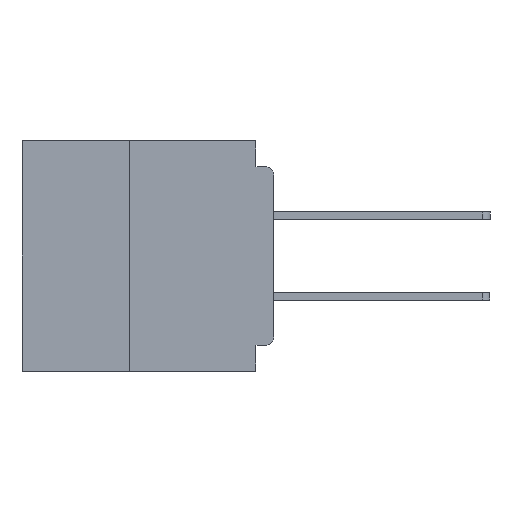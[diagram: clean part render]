
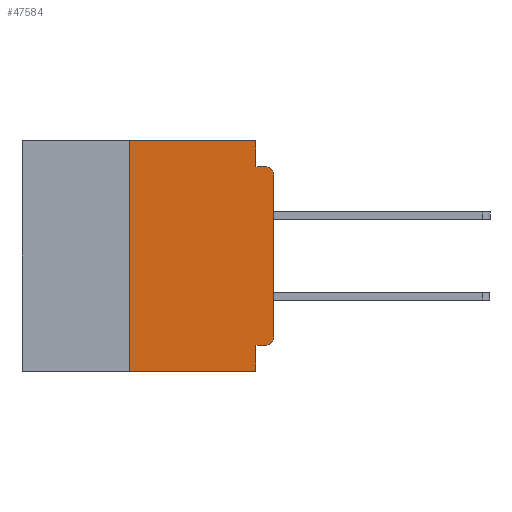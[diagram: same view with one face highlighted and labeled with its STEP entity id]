
A CAD part, left-side view. The second image highlights one B-rep face of the part: STEP entity #47584.
In plain terms, the highlighted planar face has unit normal (-1, 0, 0).
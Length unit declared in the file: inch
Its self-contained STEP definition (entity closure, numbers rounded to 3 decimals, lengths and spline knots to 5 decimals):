
#551 = ORIENTED_EDGE ( 'NONE', *, *, #44348, .F. ) ;
#1354 = CARTESIAN_POINT ( 'NONE',  ( 0., 0.015, -0.355 ) ) ;
#2596 = VERTEX_POINT ( 'NONE', #42698 ) ;
#2674 = VERTEX_POINT ( 'NONE', #37434 ) ;
#3688 = DIRECTION ( 'NONE',  ( 0., 0., -1. ) ) ;
#3971 = VECTOR ( 'NONE', #14801, 39.37008 ) ;
#4765 = CARTESIAN_POINT ( 'NONE',  ( 0., 0., 0. ) ) ;
#5240 = LINE ( 'NONE', #30179, #3971 ) ;
#5600 = CARTESIAN_POINT ( 'NONE',  ( 0., 0., -0.045 ) ) ;
#5783 = DIRECTION ( 'NONE',  ( 0., -1., 0. ) ) ;
#5863 = VECTOR ( 'NONE', #9528, 39.37008 ) ;
#6211 = ORIENTED_EDGE ( 'NONE', *, *, #15123, .T. ) ;
#8148 = EDGE_CURVE ( 'NONE', #34500, #45602, #39789, .T. ) ;
#8885 = DIRECTION ( 'NONE',  ( -1., 0., 0. ) ) ;
#9216 = EDGE_LOOP ( 'NONE', ( #45382, #16766, #22929, #38155, #13139, #35107, #6211, #551, #44868, #35758 ) ) ;
#9344 = CARTESIAN_POINT ( 'NONE',  ( 0., 0., -0.355 ) ) ;
#9528 = DIRECTION ( 'NONE',  ( 0., 1., 0. ) ) ;
#11575 = VERTEX_POINT ( 'NONE', #28146 ) ;
#13139 = ORIENTED_EDGE ( 'NONE', *, *, #25126, .F. ) ;
#14038 = VECTOR ( 'NONE', #36709, 39.37008 ) ;
#14173 = DIRECTION ( 'NONE',  ( -1., 0., 0. ) ) ;
#14774 = DIRECTION ( 'NONE',  ( 0., 0., -1. ) ) ;
#14801 = DIRECTION ( 'NONE',  ( 0., 0., 1. ) ) ;
#15123 = EDGE_CURVE ( 'NONE', #2596, #48082, #33600, .T. ) ;
#15562 = VECTOR ( 'NONE', #33870, 39.37008 ) ;
#15945 = VECTOR ( 'NONE', #5783, 39.37008 ) ;
#16476 = LINE ( 'NONE', #9344, #5863 ) ;
#16766 = ORIENTED_EDGE ( 'NONE', *, *, #32309, .T. ) ;
#17312 = VERTEX_POINT ( 'NONE', #41623 ) ;
#18422 = VERTEX_POINT ( 'NONE', #25408 ) ;
#19738 = VECTOR ( 'NONE', #40047, 39.37008 ) ;
#20898 = CARTESIAN_POINT ( 'NONE',  ( 0., 0.031, -0.045 ) ) ;
#20993 = LINE ( 'NONE', #24383, #19738 ) ;
#21926 = CARTESIAN_POINT ( 'NONE',  ( 0., 0.031, -0.355 ) ) ;
#22929 = ORIENTED_EDGE ( 'NONE', *, *, #38788, .F. ) ;
#23458 = VERTEX_POINT ( 'NONE', #20898 ) ;
#24265 = CARTESIAN_POINT ( 'NONE',  ( 0., 0., -0.34 ) ) ;
#24383 = CARTESIAN_POINT ( 'NONE',  ( 0., 0.031, -0.4 ) ) ;
#25126 = EDGE_CURVE ( 'NONE', #2674, #18422, #36331, .T. ) ;
#25408 = CARTESIAN_POINT ( 'NONE',  ( 0., 0.031, 0. ) ) ;
#26416 = CARTESIAN_POINT ( 'NONE',  ( 0., 0.437, 0. ) ) ;
#27399 = CARTESIAN_POINT ( 'NONE',  ( 0., 0.031, 0. ) ) ;
#28146 = CARTESIAN_POINT ( 'NONE',  ( 0., 0.015, -0.045 ) ) ;
#28427 = DIRECTION ( 'NONE',  ( 0., 0., 1. ) ) ;
#28882 = CARTESIAN_POINT ( 'NONE',  ( 0., 0.437, -0.4 ) ) ;
#28960 = AXIS2_PLACEMENT_3D ( 'NONE', #26416, #38172, #14774 ) ;
#29856 = CIRCLE ( 'NONE', #41732, 0.015 ) ;
#29941 = CARTESIAN_POINT ( 'NONE',  ( 0., 0.437, 0. ) ) ;
#30179 = CARTESIAN_POINT ( 'NONE',  ( 0., 0.25, -0.4 ) ) ;
#30491 = AXIS2_PLACEMENT_3D ( 'NONE', #32381, #8885, #36300 ) ;
#31690 = EDGE_CURVE ( 'NONE', #34500, #32763, #16476, .T. ) ;
#32309 = EDGE_CURVE ( 'NONE', #17312, #11575, #29856, .T. ) ;
#32381 = CARTESIAN_POINT ( 'NONE',  ( 0., 0.015, -0.34 ) ) ;
#32763 = VERTEX_POINT ( 'NONE', #21926 ) ;
#33600 = LINE ( 'NONE', #28882, #14038 ) ;
#33788 = EDGE_CURVE ( 'NONE', #45602, #17312, #47873, .T. ) ;
#33870 = DIRECTION ( 'NONE',  ( 0., -1., 0. ) ) ;
#34254 = PLANE ( 'NONE',  #28960 ) ;
#34500 = VERTEX_POINT ( 'NONE', #1354 ) ;
#35107 = ORIENTED_EDGE ( 'NONE', *, *, #37750, .F. ) ;
#35758 = ORIENTED_EDGE ( 'NONE', *, *, #8148, .T. ) ;
#36300 = DIRECTION ( 'NONE',  ( 0., 0., -1. ) ) ;
#36331 = LINE ( 'NONE', #29941, #15562 ) ;
#36363 = VECTOR ( 'NONE', #28427, 39.37008 ) ;
#36709 = DIRECTION ( 'NONE',  ( 0., -1., 0. ) ) ;
#36710 = LINE ( 'NONE', #5600, #15945 ) ;
#37094 = CARTESIAN_POINT ( 'NONE',  ( 0., 0.031, -0.4 ) ) ;
#37434 = CARTESIAN_POINT ( 'NONE',  ( 0., 0.25, 0. ) ) ;
#37554 = CARTESIAN_POINT ( 'NONE',  ( 0., 0.015, -0.06 ) ) ;
#37750 = EDGE_CURVE ( 'NONE', #2596, #2674, #5240, .T. ) ;
#38155 = ORIENTED_EDGE ( 'NONE', *, *, #44805, .F. ) ;
#38172 = DIRECTION ( 'NONE',  ( 1., 0., 0. ) ) ;
#38788 = EDGE_CURVE ( 'NONE', #23458, #11575, #36710, .T. ) ;
#39789 = CIRCLE ( 'NONE', #30491, 0.015 ) ;
#40047 = DIRECTION ( 'NONE',  ( 0., 0., -1. ) ) ;
#40052 = VECTOR ( 'NONE', #3688, 39.37008 ) ;
#41488 = DIRECTION ( 'NONE',  ( 0., 0., -1. ) ) ;
#41623 = CARTESIAN_POINT ( 'NONE',  ( 0., 0., -0.06 ) ) ;
#41732 = AXIS2_PLACEMENT_3D ( 'NONE', #37554, #14173, #41488 ) ;
#42698 = CARTESIAN_POINT ( 'NONE',  ( 0., 0.25, -0.4 ) ) ;
#44348 = EDGE_CURVE ( 'NONE', #32763, #48082, #20993, .T. ) ;
#44805 = EDGE_CURVE ( 'NONE', #18422, #23458, #49068, .T. ) ;
#44868 = ORIENTED_EDGE ( 'NONE', *, *, #31690, .F. ) ;
#45382 = ORIENTED_EDGE ( 'NONE', *, *, #33788, .T. ) ;
#45602 = VERTEX_POINT ( 'NONE', #24265 ) ;
#46969 = FACE_OUTER_BOUND ( 'NONE', #9216, .T. ) ;
#47584 = ADVANCED_FACE ( 'NONE', ( #46969 ), #34254, .F. ) ;
#47873 = LINE ( 'NONE', #4765, #36363 ) ;
#48082 = VERTEX_POINT ( 'NONE', #37094 ) ;
#49068 = LINE ( 'NONE', #27399, #40052 ) ;
